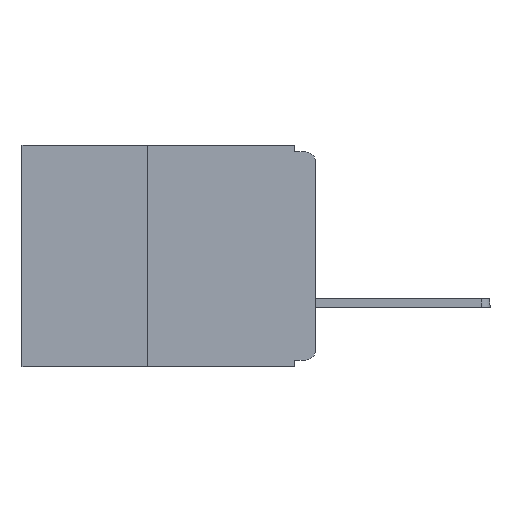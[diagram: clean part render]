
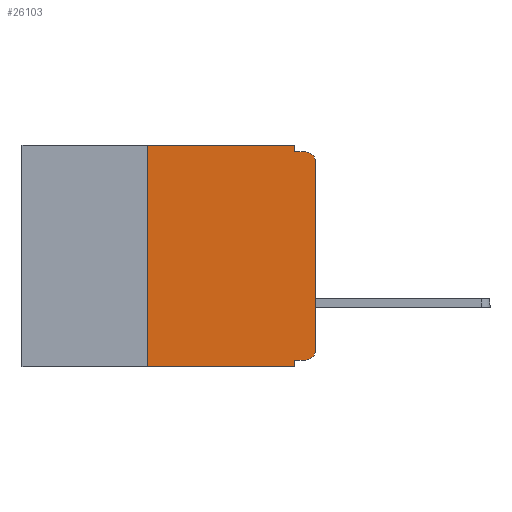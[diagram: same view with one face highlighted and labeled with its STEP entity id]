
A CAD part, left-side view. The second image highlights one B-rep face of the part: STEP entity #26103.
In plain terms, the highlighted planar face has unit normal (-1, 0, 0).
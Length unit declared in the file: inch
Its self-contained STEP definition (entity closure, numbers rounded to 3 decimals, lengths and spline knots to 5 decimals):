
#443 = VERTEX_POINT ( 'NONE', #1286 ) ;
#946 = EDGE_CURVE ( 'NONE', #13940, #7456, #29087, .T. ) ;
#1209 = DIRECTION ( 'NONE',  ( 0., 1., 0. ) ) ;
#1286 = CARTESIAN_POINT ( 'NONE',  ( 0., 0.031, -0.32 ) ) ;
#1374 = EDGE_CURVE ( 'NONE', #20289, #14172, #16401, .T. ) ;
#1465 = DIRECTION ( 'NONE',  ( -1., 0., 0. ) ) ;
#2073 = LINE ( 'NONE', #12705, #20881 ) ;
#2524 = LINE ( 'NONE', #24903, #21318 ) ;
#2680 = CARTESIAN_POINT ( 'NONE',  ( 0., 0., -0.32 ) ) ;
#2965 = ORIENTED_EDGE ( 'NONE', *, *, #946, .T. ) ;
#3009 = EDGE_CURVE ( 'NONE', #3911, #9073, #11853, .T. ) ;
#3083 = EDGE_CURVE ( 'NONE', #13940, #443, #3425, .T. ) ;
#3425 = LINE ( 'NONE', #2680, #29700 ) ;
#3911 = VERTEX_POINT ( 'NONE', #30639 ) ;
#4322 = VERTEX_POINT ( 'NONE', #18497 ) ;
#4975 = VECTOR ( 'NONE', #24630, 39.37008 ) ;
#5979 = CARTESIAN_POINT ( 'NONE',  ( 0., 0., -0.025 ) ) ;
#6696 = CARTESIAN_POINT ( 'NONE',  ( 0., 0.437, -0.33 ) ) ;
#7030 = DIRECTION ( 'NONE',  ( 0., -1., 0. ) ) ;
#7178 = EDGE_CURVE ( 'NONE', #20289, #18885, #9526, .T. ) ;
#7456 = VERTEX_POINT ( 'NONE', #22956 ) ;
#7814 = ORIENTED_EDGE ( 'NONE', *, *, #16938, .F. ) ;
#7892 = VECTOR ( 'NONE', #22011, 39.37008 ) ;
#9073 = VERTEX_POINT ( 'NONE', #32231 ) ;
#9339 = ORIENTED_EDGE ( 'NONE', *, *, #26576, .F. ) ;
#9526 = LINE ( 'NONE', #6696, #7892 ) ;
#10006 = VERTEX_POINT ( 'NONE', #5979 ) ;
#10398 = EDGE_CURVE ( 'NONE', #14172, #3911, #2073, .T. ) ;
#10975 = LINE ( 'NONE', #22076, #4975 ) ;
#11492 = CARTESIAN_POINT ( 'NONE',  ( 0., 0.25, -0.33 ) ) ;
#11853 = LINE ( 'NONE', #20668, #32051 ) ;
#12103 = ORIENTED_EDGE ( 'NONE', *, *, #15531, .T. ) ;
#12429 = CIRCLE ( 'NONE', #25947, 0.015 ) ;
#12705 = CARTESIAN_POINT ( 'NONE',  ( 0., 0.437, 0. ) ) ;
#12790 = ORIENTED_EDGE ( 'NONE', *, *, #3083, .F. ) ;
#12795 = PLANE ( 'NONE',  #22108 ) ;
#13894 = CARTESIAN_POINT ( 'NONE',  ( 0., 0.015, -0.025 ) ) ;
#13940 = VERTEX_POINT ( 'NONE', #28343 ) ;
#14172 = VERTEX_POINT ( 'NONE', #31840 ) ;
#15104 = CARTESIAN_POINT ( 'NONE',  ( 0., 0., 0. ) ) ;
#15133 = ORIENTED_EDGE ( 'NONE', *, *, #1374, .F. ) ;
#15374 = DIRECTION ( 'NONE',  ( 0., 0., -1. ) ) ;
#15531 = EDGE_CURVE ( 'NONE', #7456, #10006, #15919, .T. ) ;
#15581 = VECTOR ( 'NONE', #20613, 39.37008 ) ;
#15919 = LINE ( 'NONE', #15104, #22648 ) ;
#16401 = LINE ( 'NONE', #21047, #15581 ) ;
#16446 = DIRECTION ( 'NONE',  ( 0., 0., -1. ) ) ;
#16938 = EDGE_CURVE ( 'NONE', #443, #18885, #10975, .T. ) ;
#17007 = FACE_OUTER_BOUND ( 'NONE', #29690, .T. ) ;
#17790 = ORIENTED_EDGE ( 'NONE', *, *, #7178, .T. ) ;
#18206 = DIRECTION ( 'NONE',  ( 0., 0., -1. ) ) ;
#18497 = CARTESIAN_POINT ( 'NONE',  ( 0., 0.015, -0.01 ) ) ;
#18885 = VERTEX_POINT ( 'NONE', #20110 ) ;
#20110 = CARTESIAN_POINT ( 'NONE',  ( 0., 0.031, -0.33 ) ) ;
#20289 = VERTEX_POINT ( 'NONE', #11492 ) ;
#20405 = CARTESIAN_POINT ( 'NONE',  ( 0., 0.437, 0. ) ) ;
#20425 = DIRECTION ( 'NONE',  ( 0., -1., 0. ) ) ;
#20613 = DIRECTION ( 'NONE',  ( 0., 0., 1. ) ) ;
#20668 = CARTESIAN_POINT ( 'NONE',  ( 0., 0.031, 0. ) ) ;
#20881 = VECTOR ( 'NONE', #20425, 39.37008 ) ;
#20958 = AXIS2_PLACEMENT_3D ( 'NONE', #31721, #1465, #31932 ) ;
#21047 = CARTESIAN_POINT ( 'NONE',  ( 0., 0.25, -0.33 ) ) ;
#21318 = VECTOR ( 'NONE', #7030, 39.37008 ) ;
#22011 = DIRECTION ( 'NONE',  ( 0., -1., 0. ) ) ;
#22076 = CARTESIAN_POINT ( 'NONE',  ( 0., 0.031, -0.33 ) ) ;
#22108 = AXIS2_PLACEMENT_3D ( 'NONE', #20405, #30501, #15374 ) ;
#22648 = VECTOR ( 'NONE', #25200, 39.37008 ) ;
#22956 = CARTESIAN_POINT ( 'NONE',  ( 0., 0., -0.305 ) ) ;
#24562 = ORIENTED_EDGE ( 'NONE', *, *, #10398, .F. ) ;
#24630 = DIRECTION ( 'NONE',  ( 0., 0., -1. ) ) ;
#24903 = CARTESIAN_POINT ( 'NONE',  ( 0., 0., -0.01 ) ) ;
#25139 = ORIENTED_EDGE ( 'NONE', *, *, #28142, .T. ) ;
#25200 = DIRECTION ( 'NONE',  ( 0., 0., 1. ) ) ;
#25947 = AXIS2_PLACEMENT_3D ( 'NONE', #13894, #31556, #16446 ) ;
#26103 = ADVANCED_FACE ( 'NONE', ( #17007 ), #12795, .F. ) ;
#26576 = EDGE_CURVE ( 'NONE', #9073, #4322, #2524, .T. ) ;
#28142 = EDGE_CURVE ( 'NONE', #10006, #4322, #12429, .T. ) ;
#28343 = CARTESIAN_POINT ( 'NONE',  ( 0., 0.015, -0.32 ) ) ;
#28973 = ORIENTED_EDGE ( 'NONE', *, *, #3009, .F. ) ;
#29087 = CIRCLE ( 'NONE', #20958, 0.015 ) ;
#29690 = EDGE_LOOP ( 'NONE', ( #12103, #25139, #9339, #28973, #24562, #15133, #17790, #7814, #12790, #2965 ) ) ;
#29700 = VECTOR ( 'NONE', #1209, 39.37008 ) ;
#30501 = DIRECTION ( 'NONE',  ( 1., 0., 0. ) ) ;
#30639 = CARTESIAN_POINT ( 'NONE',  ( 0., 0.031, 0. ) ) ;
#31556 = DIRECTION ( 'NONE',  ( -1., 0., 0. ) ) ;
#31721 = CARTESIAN_POINT ( 'NONE',  ( 0., 0.015, -0.305 ) ) ;
#31840 = CARTESIAN_POINT ( 'NONE',  ( 0., 0.25, 0. ) ) ;
#31932 = DIRECTION ( 'NONE',  ( 0., 0., -1. ) ) ;
#32051 = VECTOR ( 'NONE', #18206, 39.37008 ) ;
#32231 = CARTESIAN_POINT ( 'NONE',  ( 0., 0.031, -0.01 ) ) ;
